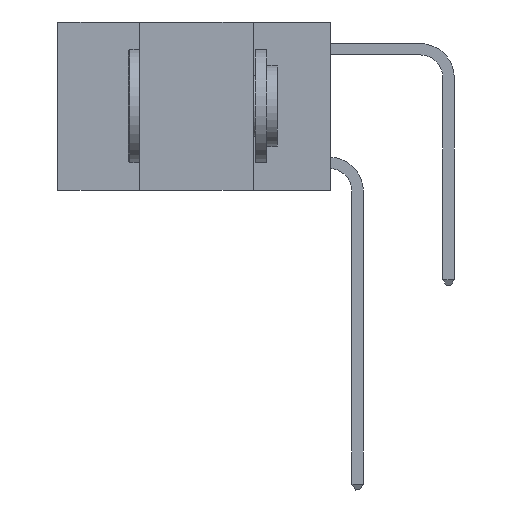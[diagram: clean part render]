
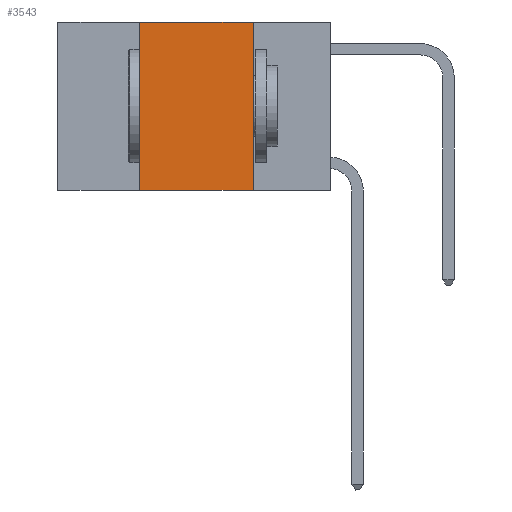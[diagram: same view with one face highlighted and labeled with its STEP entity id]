
A CAD part, left-side view. The second image highlights one B-rep face of the part: STEP entity #3543.
In plain terms, the highlighted planar face has unit normal (-1, 0, 0).
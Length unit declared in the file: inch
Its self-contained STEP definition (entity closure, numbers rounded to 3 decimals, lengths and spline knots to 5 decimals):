
#1740 = EDGE_CURVE ( 'NONE', #18711, #7925, #15804, .T. ) ;
#1742 = VERTEX_POINT ( 'NONE', #19688 ) ;
#3150 = VECTOR ( 'NONE', #17491, 39.37008 ) ;
#3543 = ADVANCED_FACE ( 'NONE', ( #5004 ), #18883, .F. ) ;
#4213 = VECTOR ( 'NONE', #4936, 39.37008 ) ;
#4313 = DIRECTION ( 'NONE',  ( 1., 0., 0. ) ) ;
#4936 = DIRECTION ( 'NONE',  ( 0., 0., 1. ) ) ;
#5004 = FACE_OUTER_BOUND ( 'NONE', #30347, .T. ) ;
#5341 = CARTESIAN_POINT ( 'NONE',  ( 0., 0.6, 0. ) ) ;
#6139 = VECTOR ( 'NONE', #19939, 39.37008 ) ;
#7808 = CARTESIAN_POINT ( 'NONE',  ( 0., 0.17, 0. ) ) ;
#7903 = EDGE_CURVE ( 'NONE', #26613, #1742, #18386, .T. ) ;
#7925 = VERTEX_POINT ( 'NONE', #10229 ) ;
#8936 = AXIS2_PLACEMENT_3D ( 'NONE', #8985, #4313, #21307 ) ;
#8985 = CARTESIAN_POINT ( 'NONE',  ( 0., 0.6, 0. ) ) ;
#9098 = ORIENTED_EDGE ( 'NONE', *, *, #16487, .F. ) ;
#10229 = CARTESIAN_POINT ( 'NONE',  ( 0., 0.17, -0.37 ) ) ;
#10678 = LINE ( 'NONE', #29219, #4213 ) ;
#10853 = VECTOR ( 'NONE', #17277, 39.37008 ) ;
#14366 = ORIENTED_EDGE ( 'NONE', *, *, #1740, .T. ) ;
#15804 = LINE ( 'NONE', #29409, #10853 ) ;
#16487 = EDGE_CURVE ( 'NONE', #18711, #26613, #10678, .T. ) ;
#17277 = DIRECTION ( 'NONE',  ( 0., -1., 0. ) ) ;
#17491 = DIRECTION ( 'NONE',  ( 0., -1., 0. ) ) ;
#17534 = CARTESIAN_POINT ( 'NONE',  ( 0., 0.42, 0. ) ) ;
#18010 = ORIENTED_EDGE ( 'NONE', *, *, #31002, .F. ) ;
#18335 = CARTESIAN_POINT ( 'NONE',  ( 0., 0.42, -0.37 ) ) ;
#18386 = LINE ( 'NONE', #5341, #3150 ) ;
#18711 = VERTEX_POINT ( 'NONE', #18335 ) ;
#18883 = PLANE ( 'NONE',  #8936 ) ;
#19688 = CARTESIAN_POINT ( 'NONE',  ( 0., 0.17, 0. ) ) ;
#19939 = DIRECTION ( 'NONE',  ( 0., 0., -1. ) ) ;
#21307 = DIRECTION ( 'NONE',  ( 0., 0., -1. ) ) ;
#22899 = ORIENTED_EDGE ( 'NONE', *, *, #7903, .F. ) ;
#25569 = LINE ( 'NONE', #7808, #6139 ) ;
#26613 = VERTEX_POINT ( 'NONE', #17534 ) ;
#29219 = CARTESIAN_POINT ( 'NONE',  ( 0., 0.42, 0. ) ) ;
#29409 = CARTESIAN_POINT ( 'NONE',  ( 0., 0.6, -0.37 ) ) ;
#30347 = EDGE_LOOP ( 'NONE', ( #18010, #22899, #9098, #14366 ) ) ;
#31002 = EDGE_CURVE ( 'NONE', #1742, #7925, #25569, .T. ) ;
